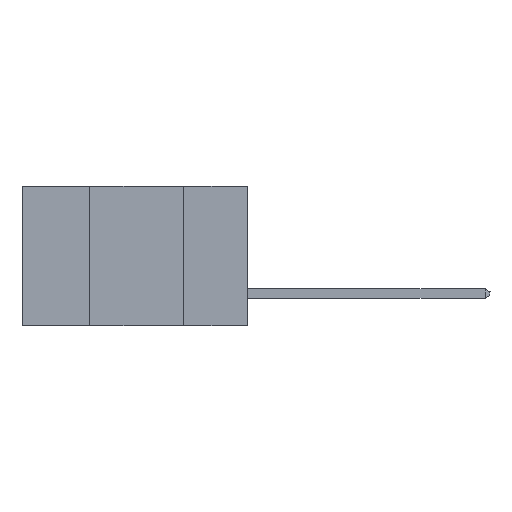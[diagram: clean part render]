
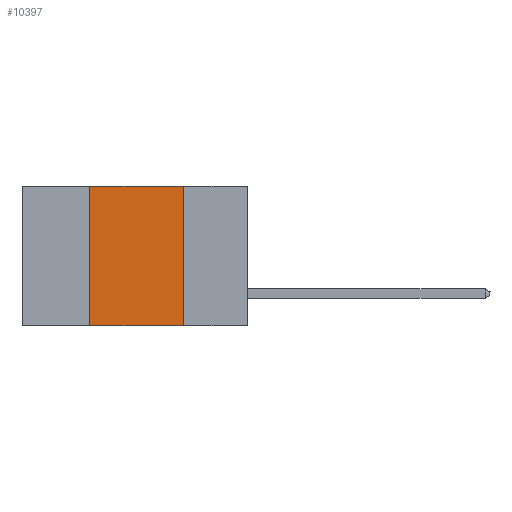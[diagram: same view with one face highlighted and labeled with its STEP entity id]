
A CAD part, left-side view. The second image highlights one B-rep face of the part: STEP entity #10397.
In plain terms, the highlighted planar face has unit normal (-1, 0, 0).
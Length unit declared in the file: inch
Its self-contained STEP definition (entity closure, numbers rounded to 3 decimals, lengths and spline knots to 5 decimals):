
#544 = VERTEX_POINT ( 'NONE', #18356 ) ;
#614 = CARTESIAN_POINT ( 'NONE',  ( 0., 0.42, 0. ) ) ;
#775 = VECTOR ( 'NONE', #3695, 39.37008 ) ;
#1046 = VERTEX_POINT ( 'NONE', #12066 ) ;
#1206 = EDGE_CURVE ( 'NONE', #5606, #1046, #9305, .T. ) ;
#1244 = CARTESIAN_POINT ( 'NONE',  ( 0., 0.42, -0.37 ) ) ;
#1890 = DIRECTION ( 'NONE',  ( 0., -1., 0. ) ) ;
#2250 = CARTESIAN_POINT ( 'NONE',  ( 0., 0.17, -0.37 ) ) ;
#2350 = DIRECTION ( 'NONE',  ( 0., 0., -1. ) ) ;
#3695 = DIRECTION ( 'NONE',  ( 0., 0., 1. ) ) ;
#3794 = LINE ( 'NONE', #17261, #775 ) ;
#4093 = ORIENTED_EDGE ( 'NONE', *, *, #1206, .T. ) ;
#4493 = EDGE_CURVE ( 'NONE', #5606, #15557, #3794, .T. ) ;
#4895 = FACE_OUTER_BOUND ( 'NONE', #5173, .T. ) ;
#5173 = EDGE_LOOP ( 'NONE', ( #6344, #16704, #15651, #4093 ) ) ;
#5227 = VECTOR ( 'NONE', #16127, 39.37008 ) ;
#5606 = VERTEX_POINT ( 'NONE', #1244 ) ;
#5917 = CARTESIAN_POINT ( 'NONE',  ( 0., 0.6, 0. ) ) ;
#6344 = ORIENTED_EDGE ( 'NONE', *, *, #16464, .F. ) ;
#7172 = EDGE_CURVE ( 'NONE', #15557, #544, #11743, .T. ) ;
#7774 = DIRECTION ( 'NONE',  ( 1., 0., 0. ) ) ;
#9305 = LINE ( 'NONE', #15441, #15606 ) ;
#10397 = ADVANCED_FACE ( 'NONE', ( #4895 ), #15482, .F. ) ;
#11007 = CARTESIAN_POINT ( 'NONE',  ( 0., 0.6, 0. ) ) ;
#11103 = VECTOR ( 'NONE', #2350, 39.37008 ) ;
#11743 = LINE ( 'NONE', #5917, #5227 ) ;
#12066 = CARTESIAN_POINT ( 'NONE',  ( 0., 0.17, -0.37 ) ) ;
#12906 = LINE ( 'NONE', #2250, #11103 ) ;
#15441 = CARTESIAN_POINT ( 'NONE',  ( 0., 0.6, -0.37 ) ) ;
#15482 = PLANE ( 'NONE',  #19219 ) ;
#15557 = VERTEX_POINT ( 'NONE', #614 ) ;
#15606 = VECTOR ( 'NONE', #1890, 39.37008 ) ;
#15651 = ORIENTED_EDGE ( 'NONE', *, *, #4493, .F. ) ;
#16127 = DIRECTION ( 'NONE',  ( 0., -1., 0. ) ) ;
#16464 = EDGE_CURVE ( 'NONE', #544, #1046, #12906, .T. ) ;
#16704 = ORIENTED_EDGE ( 'NONE', *, *, #7172, .F. ) ;
#17169 = DIRECTION ( 'NONE',  ( 0., 0., -1. ) ) ;
#17261 = CARTESIAN_POINT ( 'NONE',  ( 0., 0.42, -0.37 ) ) ;
#18356 = CARTESIAN_POINT ( 'NONE',  ( 0., 0.17, 0. ) ) ;
#19219 = AXIS2_PLACEMENT_3D ( 'NONE', #11007, #7774, #17169 ) ;
